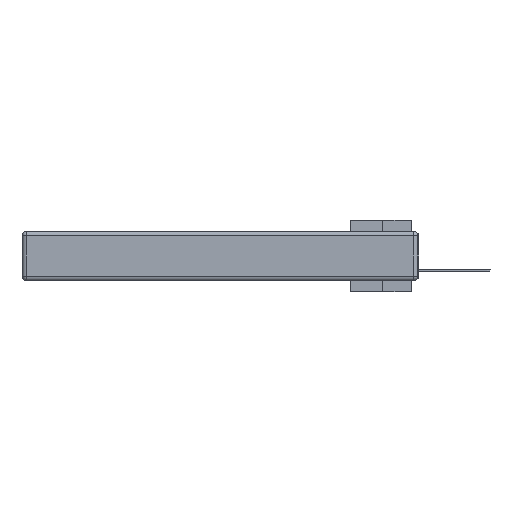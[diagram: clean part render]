
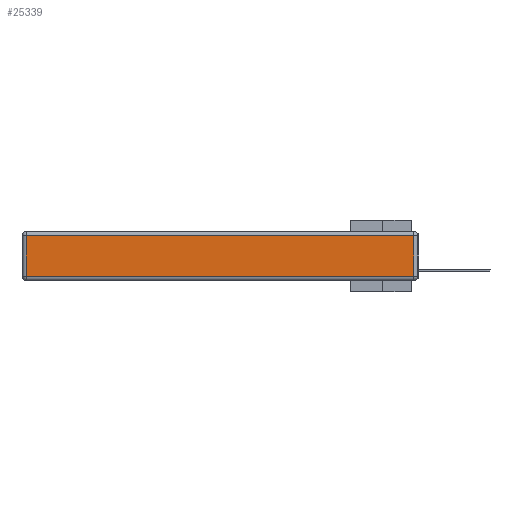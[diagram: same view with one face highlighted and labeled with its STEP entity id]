
A CAD part, left-side view. The second image highlights one B-rep face of the part: STEP entity #25339.
In plain terms, the highlighted planar face has unit normal (-1, 0, 0).
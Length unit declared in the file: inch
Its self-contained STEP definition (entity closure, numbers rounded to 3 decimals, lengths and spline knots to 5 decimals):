
#546 = CARTESIAN_POINT ( 'NONE',  ( 0., 0.03, -0.03 ) ) ;
#990 = CARTESIAN_POINT ( 'NONE',  ( 0., 0., -0.343 ) ) ;
#3562 = DIRECTION ( 'NONE',  ( -1., 0., 0. ) ) ;
#4066 = LINE ( 'NONE', #18477, #24362 ) ;
#7413 = DIRECTION ( 'NONE',  ( 0., 0., 1. ) ) ;
#7843 = VERTEX_POINT ( 'NONE', #546 ) ;
#8441 = CARTESIAN_POINT ( 'NONE',  ( 0., 2.72, -0.313 ) ) ;
#8811 = EDGE_CURVE ( 'NONE', #14013, #32895, #14970, .T. ) ;
#11555 = DIRECTION ( 'NONE',  ( 0., 0., -1. ) ) ;
#13055 = LINE ( 'NONE', #26584, #35085 ) ;
#13702 = VECTOR ( 'NONE', #27738, 39.37008 ) ;
#14013 = VERTEX_POINT ( 'NONE', #8441 ) ;
#14970 = LINE ( 'NONE', #35810, #13702 ) ;
#15502 = EDGE_CURVE ( 'NONE', #32895, #7843, #13055, .T. ) ;
#17751 = ORIENTED_EDGE ( 'NONE', *, *, #15502, .T. ) ;
#17786 = PLANE ( 'NONE',  #21466 ) ;
#18133 = CARTESIAN_POINT ( 'NONE',  ( 0., 0.03, -0.313 ) ) ;
#18477 = CARTESIAN_POINT ( 'NONE',  ( 0., 2.72, -0.343 ) ) ;
#19808 = CARTESIAN_POINT ( 'NONE',  ( 0., 2.75, -0.03 ) ) ;
#21466 = AXIS2_PLACEMENT_3D ( 'NONE', #990, #3562, #33948 ) ;
#21782 = ORIENTED_EDGE ( 'NONE', *, *, #8811, .T. ) ;
#22642 = VERTEX_POINT ( 'NONE', #35635 ) ;
#22762 = EDGE_CURVE ( 'NONE', #7843, #22642, #24061, .T. ) ;
#23192 = VECTOR ( 'NONE', #33912, 39.37008 ) ;
#24061 = LINE ( 'NONE', #19808, #23192 ) ;
#24362 = VECTOR ( 'NONE', #11555, 39.37008 ) ;
#25339 = ADVANCED_FACE ( 'NONE', ( #32843 ), #17786, .T. ) ;
#25666 = ORIENTED_EDGE ( 'NONE', *, *, #22762, .T. ) ;
#26584 = CARTESIAN_POINT ( 'NONE',  ( 0., 0.03, -0.343 ) ) ;
#26925 = EDGE_LOOP ( 'NONE', ( #21782, #17751, #25666, #33366 ) ) ;
#27738 = DIRECTION ( 'NONE',  ( 0., -1., 0. ) ) ;
#28160 = EDGE_CURVE ( 'NONE', #22642, #14013, #4066, .T. ) ;
#32843 = FACE_OUTER_BOUND ( 'NONE', #26925, .T. ) ;
#32895 = VERTEX_POINT ( 'NONE', #18133 ) ;
#33366 = ORIENTED_EDGE ( 'NONE', *, *, #28160, .T. ) ;
#33912 = DIRECTION ( 'NONE',  ( 0., 1., 0. ) ) ;
#33948 = DIRECTION ( 'NONE',  ( 0., 0., 1. ) ) ;
#35085 = VECTOR ( 'NONE', #7413, 39.37008 ) ;
#35635 = CARTESIAN_POINT ( 'NONE',  ( 0., 2.72, -0.03 ) ) ;
#35810 = CARTESIAN_POINT ( 'NONE',  ( 0., 0., -0.313 ) ) ;
